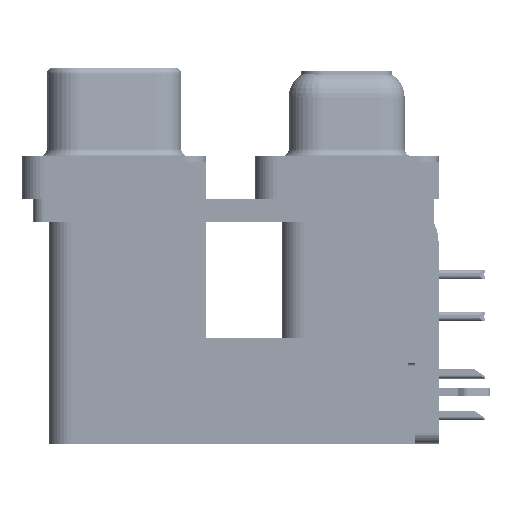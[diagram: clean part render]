
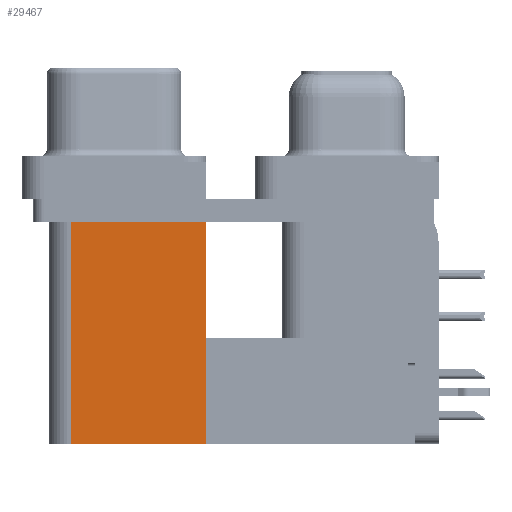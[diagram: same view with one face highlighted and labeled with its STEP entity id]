
A CAD part, left-side view. The second image highlights one B-rep face of the part: STEP entity #29467.
In plain terms, the highlighted planar face has unit normal (-1, 0, 0).
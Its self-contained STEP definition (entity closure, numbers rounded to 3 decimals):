
#714 = CARTESIAN_POINT ( 'NONE',  ( 3.79, 18.8, -19.2 ) ) ;
#5238 = EDGE_CURVE ( 'NONE', #53893, #33884, #60532, .T. ) ;
#7739 = DIRECTION ( 'NONE',  ( 0., 1., 0. ) ) ;
#10574 = LINE ( 'NONE', #714, #53830 ) ;
#10737 = EDGE_LOOP ( 'NONE', ( #22532, #63380, #63817, #32862 ) ) ;
#12151 = CARTESIAN_POINT ( 'NONE',  ( 3.79, 9.6, -19.2 ) ) ;
#12815 = CARTESIAN_POINT ( 'NONE',  ( 3.79, 18.8, -2.5 ) ) ;
#13495 = CARTESIAN_POINT ( 'NONE',  ( 3.79, 9.6, -19.2 ) ) ;
#14709 = LINE ( 'NONE', #67007, #16253 ) ;
#15029 = DIRECTION ( 'NONE',  ( 0., 0., 1. ) ) ;
#16253 = VECTOR ( 'NONE', #15029, 1000. ) ;
#18506 = CARTESIAN_POINT ( 'NONE',  ( 3.79, 9.6, -2.5 ) ) ;
#19263 = VERTEX_POINT ( 'NONE', #36275 ) ;
#22532 = ORIENTED_EDGE ( 'NONE', *, *, #5238, .T. ) ;
#27768 = LINE ( 'NONE', #12151, #58341 ) ;
#29467 = ADVANCED_FACE ( 'NONE', ( #44208 ), #33661, .F. ) ;
#29595 = DIRECTION ( 'NONE',  ( 0., 1., 0. ) ) ;
#32862 = ORIENTED_EDGE ( 'NONE', *, *, #65987, .T. ) ;
#33661 = PLANE ( 'NONE',  #54566 ) ;
#33884 = VERTEX_POINT ( 'NONE', #12815 ) ;
#34979 = EDGE_CURVE ( 'NONE', #19263, #33884, #10574, .T. ) ;
#36275 = CARTESIAN_POINT ( 'NONE',  ( 3.79, 18.8, -19.2 ) ) ;
#40800 = CARTESIAN_POINT ( 'NONE',  ( 3.79, 9.6, -2.5 ) ) ;
#44208 = FACE_OUTER_BOUND ( 'NONE', #10737, .T. ) ;
#48957 = CARTESIAN_POINT ( 'NONE',  ( 3.79, 9.6, -19.2 ) ) ;
#52251 = EDGE_CURVE ( 'NONE', #56767, #19263, #27768, .T. ) ;
#53699 = VECTOR ( 'NONE', #29595, 1000. ) ;
#53830 = VECTOR ( 'NONE', #57133, 1000. ) ;
#53893 = VERTEX_POINT ( 'NONE', #18506 ) ;
#54566 = AXIS2_PLACEMENT_3D ( 'NONE', #48957, #60171, #59166 ) ;
#56767 = VERTEX_POINT ( 'NONE', #13495 ) ;
#57133 = DIRECTION ( 'NONE',  ( 0., 0., 1. ) ) ;
#58341 = VECTOR ( 'NONE', #7739, 1000. ) ;
#59166 = DIRECTION ( 'NONE',  ( 0., 0., -1. ) ) ;
#60171 = DIRECTION ( 'NONE',  ( 1., 0., 0. ) ) ;
#60532 = LINE ( 'NONE', #40800, #53699 ) ;
#63380 = ORIENTED_EDGE ( 'NONE', *, *, #34979, .F. ) ;
#63817 = ORIENTED_EDGE ( 'NONE', *, *, #52251, .F. ) ;
#65987 = EDGE_CURVE ( 'NONE', #56767, #53893, #14709, .T. ) ;
#67007 = CARTESIAN_POINT ( 'NONE',  ( 3.79, 9.6, -19.2 ) ) ;
